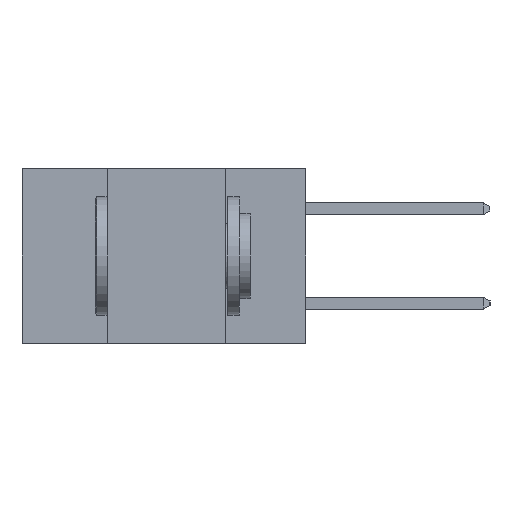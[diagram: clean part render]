
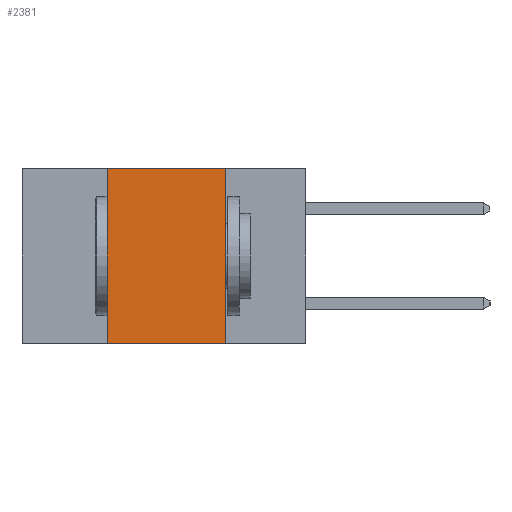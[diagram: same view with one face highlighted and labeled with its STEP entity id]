
A CAD part, left-side view. The second image highlights one B-rep face of the part: STEP entity #2381.
In plain terms, the highlighted planar face has unit normal (-1, 0, 0).
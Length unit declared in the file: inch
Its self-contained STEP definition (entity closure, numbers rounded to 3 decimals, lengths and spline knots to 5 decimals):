
#1258 = VERTEX_POINT ( 'NONE', #7390 ) ;
#2381 = ADVANCED_FACE ( 'NONE', ( #15635 ), #12713, .F. ) ;
#2420 = LINE ( 'NONE', #9565, #9288 ) ;
#2792 = ORIENTED_EDGE ( 'NONE', *, *, #10718, .F. ) ;
#2881 = EDGE_CURVE ( 'NONE', #15861, #14185, #15213, .T. ) ;
#3385 = VECTOR ( 'NONE', #11219, 39.37008 ) ;
#3417 = ORIENTED_EDGE ( 'NONE', *, *, #9887, .F. ) ;
#4074 = DIRECTION ( 'NONE',  ( 1., 0., 0. ) ) ;
#4084 = CARTESIAN_POINT ( 'NONE',  ( 0., 0.42, 0. ) ) ;
#4882 = ORIENTED_EDGE ( 'NONE', *, *, #2881, .F. ) ;
#5146 = ORIENTED_EDGE ( 'NONE', *, *, #6532, .T. ) ;
#6532 = EDGE_CURVE ( 'NONE', #15861, #6904, #8068, .T. ) ;
#6904 = VERTEX_POINT ( 'NONE', #8933 ) ;
#7390 = CARTESIAN_POINT ( 'NONE',  ( 0., 0.17, 0. ) ) ;
#7611 = DIRECTION ( 'NONE',  ( 0., 0., -1. ) ) ;
#7625 = VECTOR ( 'NONE', #11173, 39.37008 ) ;
#8068 = LINE ( 'NONE', #11967, #7625 ) ;
#8452 = VECTOR ( 'NONE', #10531, 39.37008 ) ;
#8933 = CARTESIAN_POINT ( 'NONE',  ( 0., 0.17, -0.37 ) ) ;
#9288 = VECTOR ( 'NONE', #16240, 39.37008 ) ;
#9565 = CARTESIAN_POINT ( 'NONE',  ( 0., 0.17, -0.37 ) ) ;
#9827 = CARTESIAN_POINT ( 'NONE',  ( 0., 0.6, 0. ) ) ;
#9887 = EDGE_CURVE ( 'NONE', #1258, #6904, #2420, .T. ) ;
#10390 = CARTESIAN_POINT ( 'NONE',  ( 0., 0.42, -0.37 ) ) ;
#10531 = DIRECTION ( 'NONE',  ( 0., 0., 1. ) ) ;
#10718 = EDGE_CURVE ( 'NONE', #14185, #1258, #17362, .T. ) ;
#11173 = DIRECTION ( 'NONE',  ( 0., -1., 0. ) ) ;
#11219 = DIRECTION ( 'NONE',  ( 0., -1., 0. ) ) ;
#11967 = CARTESIAN_POINT ( 'NONE',  ( 0., 0.6, -0.37 ) ) ;
#12401 = CARTESIAN_POINT ( 'NONE',  ( 0., 0.42, -0.37 ) ) ;
#12713 = PLANE ( 'NONE',  #12959 ) ;
#12959 = AXIS2_PLACEMENT_3D ( 'NONE', #15958, #4074, #7611 ) ;
#14185 = VERTEX_POINT ( 'NONE', #4084 ) ;
#15213 = LINE ( 'NONE', #10390, #8452 ) ;
#15635 = FACE_OUTER_BOUND ( 'NONE', #16208, .T. ) ;
#15861 = VERTEX_POINT ( 'NONE', #12401 ) ;
#15958 = CARTESIAN_POINT ( 'NONE',  ( 0., 0.6, 0. ) ) ;
#16208 = EDGE_LOOP ( 'NONE', ( #3417, #2792, #4882, #5146 ) ) ;
#16240 = DIRECTION ( 'NONE',  ( 0., 0., -1. ) ) ;
#17362 = LINE ( 'NONE', #9827, #3385 ) ;
